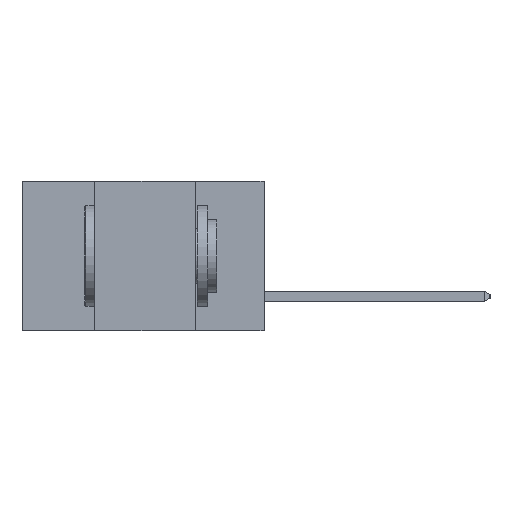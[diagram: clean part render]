
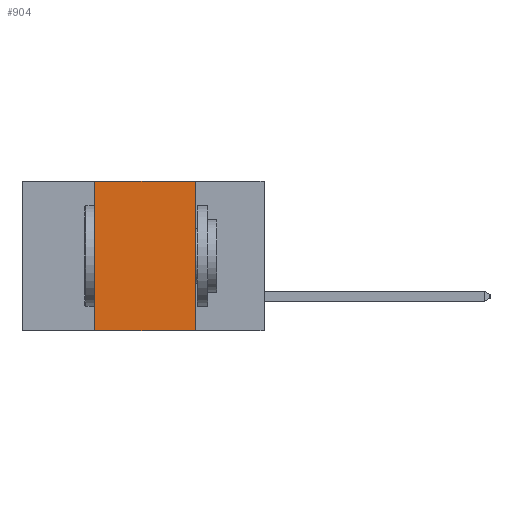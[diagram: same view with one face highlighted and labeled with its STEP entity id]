
A CAD part, left-side view. The second image highlights one B-rep face of the part: STEP entity #904.
In plain terms, the highlighted planar face has unit normal (-1, 0, 0).
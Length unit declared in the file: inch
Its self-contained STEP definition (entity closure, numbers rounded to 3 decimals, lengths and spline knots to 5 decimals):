
#201 = VERTEX_POINT ( 'NONE', #9811 ) ;
#423 = CARTESIAN_POINT ( 'NONE',  ( 0., 0.17, -0.37 ) ) ;
#486 = VECTOR ( 'NONE', #8186, 39.37008 ) ;
#904 = ADVANCED_FACE ( 'NONE', ( #9945 ), #19881, .F. ) ;
#1257 = CARTESIAN_POINT ( 'NONE',  ( 0., 0.17, -0.37 ) ) ;
#1571 = CARTESIAN_POINT ( 'NONE',  ( 0., 0.6, 0. ) ) ;
#1617 = ORIENTED_EDGE ( 'NONE', *, *, #18142, .F. ) ;
#1804 = DIRECTION ( 'NONE',  ( 0., -1., 0. ) ) ;
#3313 = AXIS2_PLACEMENT_3D ( 'NONE', #1571, #14006, #15030 ) ;
#4180 = VECTOR ( 'NONE', #9757, 39.37008 ) ;
#6371 = CARTESIAN_POINT ( 'NONE',  ( 0., 0.6, 0. ) ) ;
#6959 = DIRECTION ( 'NONE',  ( 0., 0., 1. ) ) ;
#7213 = VECTOR ( 'NONE', #6959, 39.37008 ) ;
#8186 = DIRECTION ( 'NONE',  ( 0., -1., 0. ) ) ;
#9210 = VERTEX_POINT ( 'NONE', #10145 ) ;
#9757 = DIRECTION ( 'NONE',  ( 0., 0., -1. ) ) ;
#9811 = CARTESIAN_POINT ( 'NONE',  ( 0., 0.42, 0. ) ) ;
#9945 = FACE_OUTER_BOUND ( 'NONE', #12828, .T. ) ;
#10145 = CARTESIAN_POINT ( 'NONE',  ( 0., 0.42, -0.37 ) ) ;
#12050 = ORIENTED_EDGE ( 'NONE', *, *, #16978, .F. ) ;
#12595 = ORIENTED_EDGE ( 'NONE', *, *, #15798, .F. ) ;
#12763 = VECTOR ( 'NONE', #1804, 39.37008 ) ;
#12828 = EDGE_LOOP ( 'NONE', ( #1617, #12050, #12595, #21827 ) ) ;
#13333 = LINE ( 'NONE', #19843, #12763 ) ;
#13431 = EDGE_CURVE ( 'NONE', #9210, #20109, #13333, .T. ) ;
#14006 = DIRECTION ( 'NONE',  ( 1., 0., 0. ) ) ;
#15030 = DIRECTION ( 'NONE',  ( 0., 0., -1. ) ) ;
#15798 = EDGE_CURVE ( 'NONE', #9210, #201, #16291, .T. ) ;
#16291 = LINE ( 'NONE', #19523, #7213 ) ;
#16978 = EDGE_CURVE ( 'NONE', #201, #19983, #23083, .T. ) ;
#18142 = EDGE_CURVE ( 'NONE', #19983, #20109, #18609, .T. ) ;
#18609 = LINE ( 'NONE', #423, #4180 ) ;
#19106 = CARTESIAN_POINT ( 'NONE',  ( 0., 0.17, 0. ) ) ;
#19523 = CARTESIAN_POINT ( 'NONE',  ( 0., 0.42, -0.37 ) ) ;
#19843 = CARTESIAN_POINT ( 'NONE',  ( 0., 0.6, -0.37 ) ) ;
#19881 = PLANE ( 'NONE',  #3313 ) ;
#19983 = VERTEX_POINT ( 'NONE', #19106 ) ;
#20109 = VERTEX_POINT ( 'NONE', #1257 ) ;
#21827 = ORIENTED_EDGE ( 'NONE', *, *, #13431, .T. ) ;
#23083 = LINE ( 'NONE', #6371, #486 ) ;
